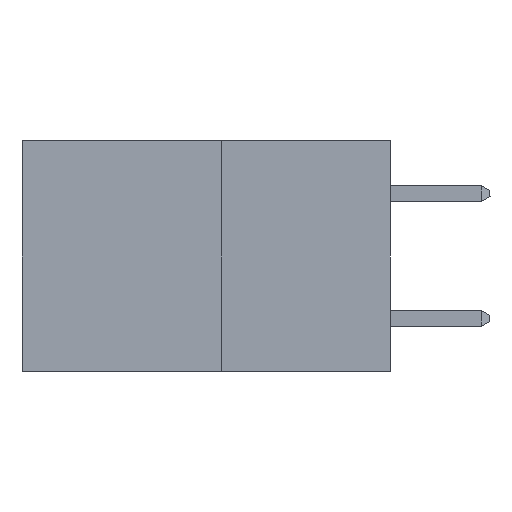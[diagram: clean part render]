
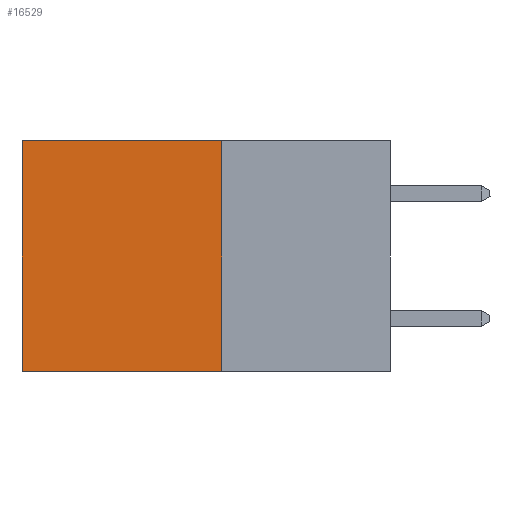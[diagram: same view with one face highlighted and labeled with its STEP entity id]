
A CAD part, left-side view. The second image highlights one B-rep face of the part: STEP entity #16529.
In plain terms, the highlighted planar face has unit normal (-1, 0, 0).
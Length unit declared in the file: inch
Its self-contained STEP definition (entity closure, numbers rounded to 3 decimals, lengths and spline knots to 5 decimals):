
#1065 = ORIENTED_EDGE ( 'NONE', *, *, #11971, .T. ) ;
#1118 = CARTESIAN_POINT ( 'NONE',  ( 0.277, 0.27, -0.37 ) ) ;
#2702 = VERTEX_POINT ( 'NONE', #1118 ) ;
#4062 = CARTESIAN_POINT ( 'NONE',  ( 0.277, 0.59, -0.37 ) ) ;
#5339 = ORIENTED_EDGE ( 'NONE', *, *, #8270, .F. ) ;
#5867 = ORIENTED_EDGE ( 'NONE', *, *, #15119, .T. ) ;
#6032 = VECTOR ( 'NONE', #13147, 39.37008 ) ;
#6773 = LINE ( 'NONE', #4062, #6032 ) ;
#6909 = DIRECTION ( 'NONE',  ( 0., 0., -1. ) ) ;
#8153 = DIRECTION ( 'NONE',  ( 1., 0., 0. ) ) ;
#8270 = EDGE_CURVE ( 'NONE', #25094, #2702, #24558, .T. ) ;
#10173 = CARTESIAN_POINT ( 'NONE',  ( 0.277, 0.27, -0.37 ) ) ;
#10341 = PLANE ( 'NONE',  #18296 ) ;
#11956 = CARTESIAN_POINT ( 'NONE',  ( 0.277, 0.59, -0.37 ) ) ;
#11971 = EDGE_CURVE ( 'NONE', #12233, #26787, #6773, .T. ) ;
#12233 = VERTEX_POINT ( 'NONE', #23061 ) ;
#12700 = FACE_OUTER_BOUND ( 'NONE', #23279, .T. ) ;
#13147 = DIRECTION ( 'NONE',  ( 0., 0., -1. ) ) ;
#13621 = DIRECTION ( 'NONE',  ( 0., 1., 0. ) ) ;
#14201 = LINE ( 'NONE', #26066, #25363 ) ;
#14630 = LINE ( 'NONE', #18021, #25785 ) ;
#15119 = EDGE_CURVE ( 'NONE', #25094, #12233, #14201, .T. ) ;
#16529 = ADVANCED_FACE ( 'NONE', ( #12700 ), #10341, .F. ) ;
#18021 = CARTESIAN_POINT ( 'NONE',  ( 0.277, 0.27, -0.37 ) ) ;
#18296 = AXIS2_PLACEMENT_3D ( 'NONE', #21678, #8153, #23917 ) ;
#18656 = VECTOR ( 'NONE', #6909, 39.37008 ) ;
#19266 = CARTESIAN_POINT ( 'NONE',  ( 0.277, 0.27, 0. ) ) ;
#21678 = CARTESIAN_POINT ( 'NONE',  ( 0.277, 0.27, -0.37 ) ) ;
#23061 = CARTESIAN_POINT ( 'NONE',  ( 0.277, 0.59, 0. ) ) ;
#23279 = EDGE_LOOP ( 'NONE', ( #1065, #27697, #5339, #5867 ) ) ;
#23917 = DIRECTION ( 'NONE',  ( 0., 0., -1. ) ) ;
#24133 = EDGE_CURVE ( 'NONE', #2702, #26787, #14630, .T. ) ;
#24558 = LINE ( 'NONE', #10173, #18656 ) ;
#25094 = VERTEX_POINT ( 'NONE', #19266 ) ;
#25363 = VECTOR ( 'NONE', #28250, 39.37008 ) ;
#25785 = VECTOR ( 'NONE', #13621, 39.37008 ) ;
#26066 = CARTESIAN_POINT ( 'NONE',  ( 0.277, 0.27, 0. ) ) ;
#26787 = VERTEX_POINT ( 'NONE', #11956 ) ;
#27697 = ORIENTED_EDGE ( 'NONE', *, *, #24133, .F. ) ;
#28250 = DIRECTION ( 'NONE',  ( 0., 1., 0. ) ) ;
